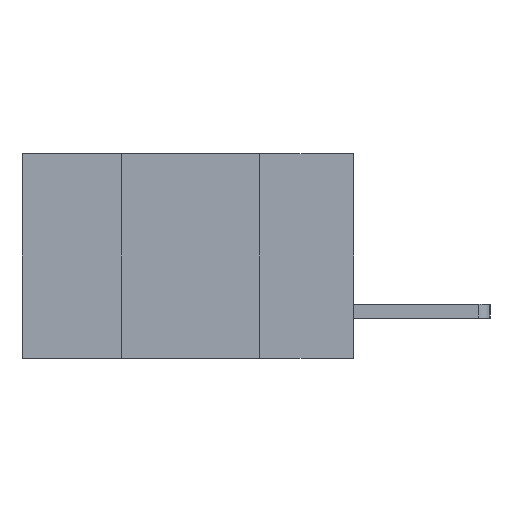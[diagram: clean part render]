
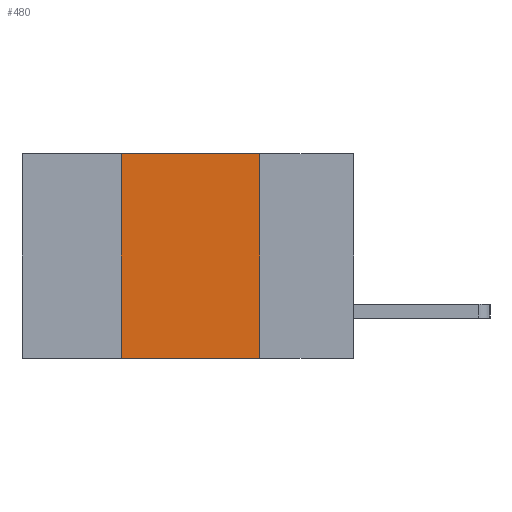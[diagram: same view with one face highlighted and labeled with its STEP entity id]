
A CAD part, left-side view. The second image highlights one B-rep face of the part: STEP entity #480.
In plain terms, the highlighted planar face has unit normal (-1, 0, 0).
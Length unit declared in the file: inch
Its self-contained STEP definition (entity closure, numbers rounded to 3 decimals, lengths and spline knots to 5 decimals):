
#104 = CARTESIAN_POINT ( 'NONE',  ( 0., 0.6, -0.37 ) ) ;
#176 = VECTOR ( 'NONE', #9434, 39.37008 ) ;
#248 = CARTESIAN_POINT ( 'NONE',  ( 0., 0.42, -0.37 ) ) ;
#480 = ADVANCED_FACE ( 'NONE', ( #10977 ), #11210, .F. ) ;
#522 = DIRECTION ( 'NONE',  ( 0., 0., -1. ) ) ;
#1506 = EDGE_CURVE ( 'NONE', #4594, #6220, #15205, .T. ) ;
#3960 = ORIENTED_EDGE ( 'NONE', *, *, #14979, .T. ) ;
#4456 = EDGE_CURVE ( 'NONE', #6220, #4558, #4646, .T. ) ;
#4558 = VERTEX_POINT ( 'NONE', #7463 ) ;
#4594 = VERTEX_POINT ( 'NONE', #248 ) ;
#4646 = LINE ( 'NONE', #14427, #176 ) ;
#4928 = ORIENTED_EDGE ( 'NONE', *, *, #1506, .F. ) ;
#4969 = DIRECTION ( 'NONE',  ( 0., -1., 0. ) ) ;
#5266 = DIRECTION ( 'NONE',  ( 0., 0., 1. ) ) ;
#5549 = LINE ( 'NONE', #11617, #9582 ) ;
#6220 = VERTEX_POINT ( 'NONE', #13406 ) ;
#6236 = AXIS2_PLACEMENT_3D ( 'NONE', #13416, #6316, #6241 ) ;
#6241 = DIRECTION ( 'NONE',  ( 0., 0., -1. ) ) ;
#6316 = DIRECTION ( 'NONE',  ( 1., 0., 0. ) ) ;
#7076 = EDGE_CURVE ( 'NONE', #4558, #10798, #5549, .T. ) ;
#7200 = ORIENTED_EDGE ( 'NONE', *, *, #7076, .F. ) ;
#7463 = CARTESIAN_POINT ( 'NONE',  ( 0., 0.17, 0. ) ) ;
#9434 = DIRECTION ( 'NONE',  ( 0., -1., 0. ) ) ;
#9582 = VECTOR ( 'NONE', #522, 39.37008 ) ;
#10798 = VERTEX_POINT ( 'NONE', #10968 ) ;
#10873 = LINE ( 'NONE', #104, #11991 ) ;
#10968 = CARTESIAN_POINT ( 'NONE',  ( 0., 0.17, -0.37 ) ) ;
#10977 = FACE_OUTER_BOUND ( 'NONE', #14776, .T. ) ;
#11210 = PLANE ( 'NONE',  #6236 ) ;
#11617 = CARTESIAN_POINT ( 'NONE',  ( 0., 0.17, 0. ) ) ;
#11991 = VECTOR ( 'NONE', #4969, 39.37008 ) ;
#12429 = CARTESIAN_POINT ( 'NONE',  ( 0., 0.42, 0. ) ) ;
#13406 = CARTESIAN_POINT ( 'NONE',  ( 0., 0.42, 0. ) ) ;
#13416 = CARTESIAN_POINT ( 'NONE',  ( 0., 0.6, 0. ) ) ;
#14306 = VECTOR ( 'NONE', #5266, 39.37008 ) ;
#14427 = CARTESIAN_POINT ( 'NONE',  ( 0., 0.6, 0. ) ) ;
#14776 = EDGE_LOOP ( 'NONE', ( #7200, #15206, #4928, #3960 ) ) ;
#14979 = EDGE_CURVE ( 'NONE', #4594, #10798, #10873, .T. ) ;
#15205 = LINE ( 'NONE', #12429, #14306 ) ;
#15206 = ORIENTED_EDGE ( 'NONE', *, *, #4456, .F. ) ;
